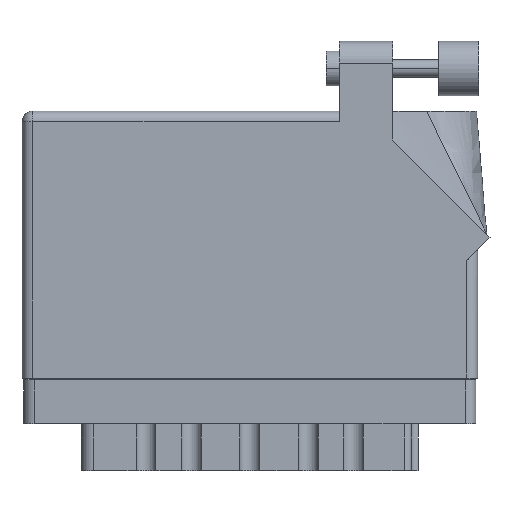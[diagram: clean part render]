
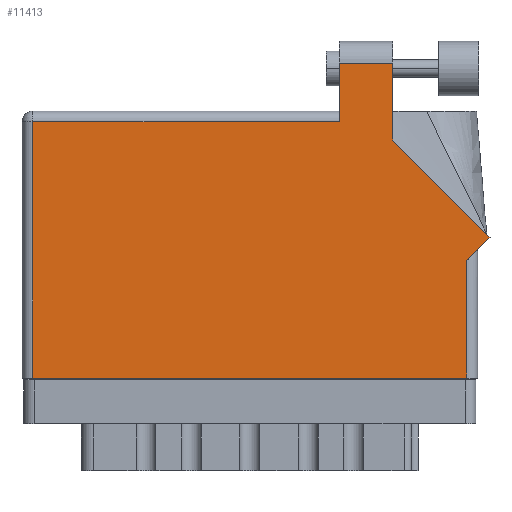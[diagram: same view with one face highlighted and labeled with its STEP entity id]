
A CAD part, front view. The second image highlights one B-rep face of the part: STEP entity #11413.
In plain terms, the highlighted face is planar.
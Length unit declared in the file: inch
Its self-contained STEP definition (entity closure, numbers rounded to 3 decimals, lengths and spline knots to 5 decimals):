
#1747 = LINE ( 'NONE', #45918, #44374 ) ;
#2099 = CARTESIAN_POINT ( 'NONE',  ( 1.819, 1.468, 0. ) ) ;
#2772 = VECTOR ( 'NONE', #18914, 39.37008 ) ;
#3729 = ORIENTED_EDGE ( 'NONE', *, *, #15554, .T. ) ;
#4549 = AXIS2_PLACEMENT_3D ( 'NONE', #30258, #30606, #17675 ) ;
#4774 = ORIENTED_EDGE ( 'NONE', *, *, #23513, .T. ) ;
#5066 = ORIENTED_EDGE ( 'NONE', *, *, #10853, .T. ) ;
#5177 = PLANE ( 'NONE',  #4549 ) ;
#6334 = CARTESIAN_POINT ( 'NONE',  ( 2.68271, 0.80771, 0. ) ) ;
#7231 = CARTESIAN_POINT ( 'NONE',  ( 0.062, 0., 0. ) ) ;
#8749 = CARTESIAN_POINT ( 'NONE',  ( 2.126, 1.36442, 0. ) ) ;
#10036 = ORIENTED_EDGE ( 'NONE', *, *, #31165, .T. ) ;
#10294 = DIRECTION ( 'NONE',  ( -1., 0., 0. ) ) ;
#10853 = EDGE_CURVE ( 'NONE', #31890, #15844, #41544, .T. ) ;
#11413 = ADVANCED_FACE ( 'NONE', ( #49921 ), #5177, .F. ) ;
#11665 = CARTESIAN_POINT ( 'NONE',  ( 2.126, 1.805, 0. ) ) ;
#12042 = CARTESIAN_POINT ( 'NONE',  ( 0.062, 0., 0. ) ) ;
#13293 = VECTOR ( 'NONE', #48984, 39.37008 ) ;
#14327 = ORIENTED_EDGE ( 'NONE', *, *, #14927, .T. ) ;
#14927 = EDGE_CURVE ( 'NONE', #23360, #17690, #15421, .T. ) ;
#15421 = LINE ( 'NONE', #8749, #24457 ) ;
#15554 = EDGE_CURVE ( 'NONE', #41498, #31890, #1747, .T. ) ;
#15844 = VERTEX_POINT ( 'NONE', #39012 ) ;
#17107 = DIRECTION ( 'NONE',  ( 0., 1., 0. ) ) ;
#17675 = DIRECTION ( 'NONE',  ( -1., 0., 0. ) ) ;
#17690 = VERTEX_POINT ( 'NONE', #11665 ) ;
#18457 = LINE ( 'NONE', #39720, #42986 ) ;
#18591 = VECTOR ( 'NONE', #24326, 39.37008 ) ;
#18649 = ORIENTED_EDGE ( 'NONE', *, *, #27312, .T. ) ;
#18914 = DIRECTION ( 'NONE',  ( 1., 0., 0. ) ) ;
#21404 = LINE ( 'NONE', #6334, #52501 ) ;
#21410 = VECTOR ( 'NONE', #10294, 39.37008 ) ;
#23360 = VERTEX_POINT ( 'NONE', #42815 ) ;
#23490 = DIRECTION ( 'NONE',  ( -0.707, 0.707, 0. ) ) ;
#23513 = EDGE_CURVE ( 'NONE', #23916, #23360, #21404, .T. ) ;
#23916 = VERTEX_POINT ( 'NONE', #33760 ) ;
#24326 = DIRECTION ( 'NONE',  ( 0.707, 0.707, 0. ) ) ;
#24457 = VECTOR ( 'NONE', #17107, 39.37008 ) ;
#25570 = LINE ( 'NONE', #7231, #13293 ) ;
#26516 = ORIENTED_EDGE ( 'NONE', *, *, #34626, .T. ) ;
#27312 = EDGE_CURVE ( 'NONE', #15844, #45216, #25570, .T. ) ;
#28319 = CARTESIAN_POINT ( 'NONE',  ( 2.612, 0.737, 0. ) ) ;
#30258 = CARTESIAN_POINT ( 'NONE',  ( 0., 1.53, 0. ) ) ;
#30269 = CARTESIAN_POINT ( 'NONE',  ( 2.55, 0.675, 0. ) ) ;
#30336 = CARTESIAN_POINT ( 'NONE',  ( 1.819, 1.805, 0. ) ) ;
#30606 = DIRECTION ( 'NONE',  ( 0., 0., -1. ) ) ;
#31165 = EDGE_CURVE ( 'NONE', #52296, #46716, #18457, .T. ) ;
#31890 = VERTEX_POINT ( 'NONE', #2099 ) ;
#32410 = LINE ( 'NONE', #30336, #21410 ) ;
#33760 = CARTESIAN_POINT ( 'NONE',  ( 2.68271, 0.80771, 0. ) ) ;
#33808 = ORIENTED_EDGE ( 'NONE', *, *, #43263, .T. ) ;
#33889 = EDGE_CURVE ( 'NONE', #17690, #41498, #32410, .T. ) ;
#34560 = ORIENTED_EDGE ( 'NONE', *, *, #33889, .T. ) ;
#34626 = EDGE_CURVE ( 'NONE', #45216, #52296, #38322, .T. ) ;
#35217 = EDGE_LOOP ( 'NONE', ( #14327, #34560, #3729, #5066, #18649, #26516, #10036, #33808, #4774 ) ) ;
#35694 = CARTESIAN_POINT ( 'NONE',  ( 0., 0., 0. ) ) ;
#37655 = VECTOR ( 'NONE', #51130, 39.37008 ) ;
#38322 = LINE ( 'NONE', #35694, #2772 ) ;
#39012 = CARTESIAN_POINT ( 'NONE',  ( 0.062, 1.468, 0. ) ) ;
#39720 = CARTESIAN_POINT ( 'NONE',  ( 2.55, 0.737, 0. ) ) ;
#39939 = LINE ( 'NONE', #28319, #18591 ) ;
#40067 = DIRECTION ( 'NONE',  ( 0., 1., 0. ) ) ;
#40189 = CARTESIAN_POINT ( 'NONE',  ( 2.55, 0., 0. ) ) ;
#41310 = CARTESIAN_POINT ( 'NONE',  ( 1.819, 1.805, 0. ) ) ;
#41498 = VERTEX_POINT ( 'NONE', #41310 ) ;
#41544 = LINE ( 'NONE', #51315, #37655 ) ;
#42815 = CARTESIAN_POINT ( 'NONE',  ( 2.126, 1.36442, 0. ) ) ;
#42986 = VECTOR ( 'NONE', #40067, 39.37008 ) ;
#43263 = EDGE_CURVE ( 'NONE', #46716, #23916, #39939, .T. ) ;
#44374 = VECTOR ( 'NONE', #50083, 39.37008 ) ;
#45216 = VERTEX_POINT ( 'NONE', #12042 ) ;
#45918 = CARTESIAN_POINT ( 'NONE',  ( 1.819, 1.53, 0. ) ) ;
#46716 = VERTEX_POINT ( 'NONE', #30269 ) ;
#48984 = DIRECTION ( 'NONE',  ( 0., -1., 0. ) ) ;
#49921 = FACE_OUTER_BOUND ( 'NONE', #35217, .T. ) ;
#50083 = DIRECTION ( 'NONE',  ( 0., -1., 0. ) ) ;
#51130 = DIRECTION ( 'NONE',  ( -1., 0., 0. ) ) ;
#51315 = CARTESIAN_POINT ( 'NONE',  ( 0., 1.468, 0. ) ) ;
#52296 = VERTEX_POINT ( 'NONE', #40189 ) ;
#52501 = VECTOR ( 'NONE', #23490, 39.37008 ) ;
